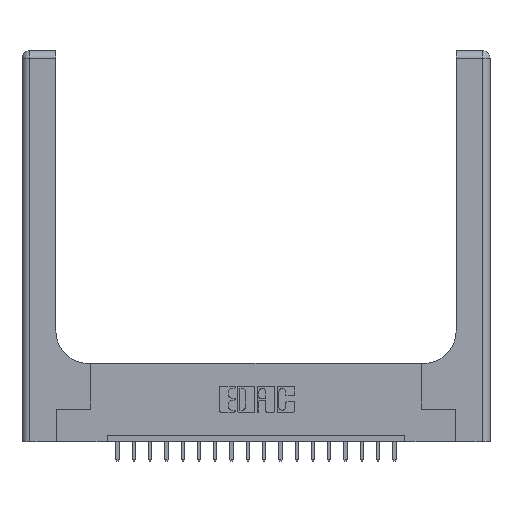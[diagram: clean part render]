
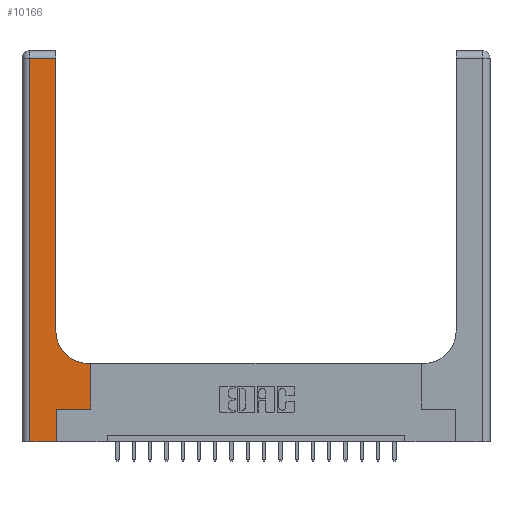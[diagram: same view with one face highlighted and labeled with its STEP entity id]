
A CAD part, top view. The second image highlights one B-rep face of the part: STEP entity #10166.
In plain terms, the highlighted planar face has unit normal (0, 0, 1).
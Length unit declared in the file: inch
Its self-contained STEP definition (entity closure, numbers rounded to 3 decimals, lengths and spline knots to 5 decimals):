
#384 = DIRECTION ( 'NONE',  ( 0., 1., 0. ) ) ;
#823 = LINE ( 'NONE', #3670, #6425 ) ;
#909 = VECTOR ( 'NONE', #10281, 39.37008 ) ;
#954 = VERTEX_POINT ( 'NONE', #8094 ) ;
#1071 = ORIENTED_EDGE ( 'NONE', *, *, #17597, .T. ) ;
#1357 = VERTEX_POINT ( 'NONE', #17571 ) ;
#1526 = DIRECTION ( 'NONE',  ( 0., 1., 0. ) ) ;
#1583 = EDGE_CURVE ( 'NONE', #9866, #954, #17144, .T. ) ;
#2341 = CARTESIAN_POINT ( 'NONE',  ( 0.265, 0., 0.37 ) ) ;
#2344 = CARTESIAN_POINT ( 'NONE',  ( 0., 3., 0.37 ) ) ;
#2351 = CARTESIAN_POINT ( 'NONE',  ( 0.265, 0.25, 0.37 ) ) ;
#2394 = EDGE_CURVE ( 'NONE', #7478, #14368, #14284, .T. ) ;
#2908 = VERTEX_POINT ( 'NONE', #2341 ) ;
#3172 = CARTESIAN_POINT ( 'NONE',  ( 0.26, 0.6, 0.37 ) ) ;
#3195 = EDGE_CURVE ( 'NONE', #14368, #14114, #9424, .T. ) ;
#3280 = DIRECTION ( 'NONE',  ( 1., 0., 0. ) ) ;
#3456 = DIRECTION ( 'NONE',  ( 0., -1., 0. ) ) ;
#3670 = CARTESIAN_POINT ( 'NONE',  ( 0., 0., 0.37 ) ) ;
#4642 = VECTOR ( 'NONE', #384, 39.37008 ) ;
#4675 = DIRECTION ( 'NONE',  ( -1., 0., 0. ) ) ;
#4888 = ORIENTED_EDGE ( 'NONE', *, *, #10034, .T. ) ;
#5113 = VERTEX_POINT ( 'NONE', #5620 ) ;
#5339 = CARTESIAN_POINT ( 'NONE',  ( 0.26, 2.94, 0.37 ) ) ;
#5620 = CARTESIAN_POINT ( 'NONE',  ( 0.51, 0.6, 0.37 ) ) ;
#5672 = AXIS2_PLACEMENT_3D ( 'NONE', #14998, #19952, #16596 ) ;
#6425 = VECTOR ( 'NONE', #12997, 39.37008 ) ;
#6560 = CARTESIAN_POINT ( 'NONE',  ( 0.26, 3., 0.37 ) ) ;
#7005 = DIRECTION ( 'NONE',  ( -1., 0., 0. ) ) ;
#7478 = VERTEX_POINT ( 'NONE', #5339 ) ;
#7869 = LINE ( 'NONE', #6560, #4642 ) ;
#8093 = EDGE_CURVE ( 'NONE', #954, #5113, #9139, .T. ) ;
#8094 = CARTESIAN_POINT ( 'NONE',  ( 0.528, 0.6, 0.37 ) ) ;
#8334 = FACE_OUTER_BOUND ( 'NONE', #18057, .T. ) ;
#8363 = ORIENTED_EDGE ( 'NONE', *, *, #1583, .T. ) ;
#8521 = DIRECTION ( 'NONE',  ( 0., 0., -1. ) ) ;
#9135 = ORIENTED_EDGE ( 'NONE', *, *, #2394, .T. ) ;
#9139 = LINE ( 'NONE', #3172, #18501 ) ;
#9194 = VECTOR ( 'NONE', #3456, 39.37008 ) ;
#9424 = LINE ( 'NONE', #16912, #9194 ) ;
#9866 = VERTEX_POINT ( 'NONE', #18079 ) ;
#9881 = CIRCLE ( 'NONE', #5672, 0.25 ) ;
#10034 = EDGE_CURVE ( 'NONE', #12422, #9866, #17464, .T. ) ;
#10166 = ADVANCED_FACE ( 'NONE', ( #8334 ), #17656, .F. ) ;
#10281 = DIRECTION ( 'NONE',  ( 0., 1., 0. ) ) ;
#10374 = CARTESIAN_POINT ( 'NONE',  ( 0.265, 0., 0.37 ) ) ;
#10807 = EDGE_CURVE ( 'NONE', #1357, #7478, #7869, .T. ) ;
#10817 = ORIENTED_EDGE ( 'NONE', *, *, #8093, .T. ) ;
#11271 = ORIENTED_EDGE ( 'NONE', *, *, #10807, .T. ) ;
#11945 = EDGE_CURVE ( 'NONE', #5113, #1357, #9881, .T. ) ;
#12290 = CARTESIAN_POINT ( 'NONE',  ( 0.528, 0.25, 0.37 ) ) ;
#12422 = VERTEX_POINT ( 'NONE', #2351 ) ;
#12499 = CARTESIAN_POINT ( 'NONE',  ( 0.265, 0.25, 0.37 ) ) ;
#12725 = VECTOR ( 'NONE', #16091, 39.37008 ) ;
#12997 = DIRECTION ( 'NONE',  ( 1., 0., 0. ) ) ;
#14114 = VERTEX_POINT ( 'NONE', #15203 ) ;
#14284 = LINE ( 'NONE', #15689, #12725 ) ;
#14320 = ORIENTED_EDGE ( 'NONE', *, *, #11945, .T. ) ;
#14368 = VERTEX_POINT ( 'NONE', #18431 ) ;
#14651 = LINE ( 'NONE', #10374, #909 ) ;
#14998 = CARTESIAN_POINT ( 'NONE',  ( 0.51, 0.85, 0.37 ) ) ;
#15203 = CARTESIAN_POINT ( 'NONE',  ( 0.06, 0., 0.37 ) ) ;
#15689 = CARTESIAN_POINT ( 'NONE',  ( 0., 2.94, 0.37 ) ) ;
#16091 = DIRECTION ( 'NONE',  ( -1., 0., 0. ) ) ;
#16596 = DIRECTION ( 'NONE',  ( 1., 0., 0. ) ) ;
#16912 = CARTESIAN_POINT ( 'NONE',  ( 0.06, 3., 0.37 ) ) ;
#16950 = VECTOR ( 'NONE', #1526, 39.37008 ) ;
#17038 = ORIENTED_EDGE ( 'NONE', *, *, #3195, .T. ) ;
#17144 = LINE ( 'NONE', #12290, #16950 ) ;
#17464 = LINE ( 'NONE', #12499, #19537 ) ;
#17571 = CARTESIAN_POINT ( 'NONE',  ( 0.26, 0.85, 0.37 ) ) ;
#17597 = EDGE_CURVE ( 'NONE', #14114, #2908, #823, .T. ) ;
#17656 = PLANE ( 'NONE',  #18227 ) ;
#18057 = EDGE_LOOP ( 'NONE', ( #11271, #9135, #17038, #1071, #18172, #4888, #8363, #10817, #14320 ) ) ;
#18079 = CARTESIAN_POINT ( 'NONE',  ( 0.528, 0.25, 0.37 ) ) ;
#18172 = ORIENTED_EDGE ( 'NONE', *, *, #18869, .T. ) ;
#18227 = AXIS2_PLACEMENT_3D ( 'NONE', #2344, #8521, #7005 ) ;
#18431 = CARTESIAN_POINT ( 'NONE',  ( 0.06, 2.94, 0.37 ) ) ;
#18501 = VECTOR ( 'NONE', #4675, 39.37008 ) ;
#18869 = EDGE_CURVE ( 'NONE', #2908, #12422, #14651, .T. ) ;
#19537 = VECTOR ( 'NONE', #3280, 39.37008 ) ;
#19952 = DIRECTION ( 'NONE',  ( 0., 0., -1. ) ) ;
